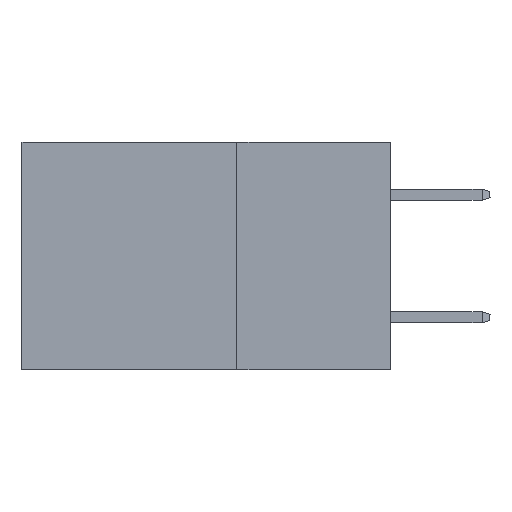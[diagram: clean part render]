
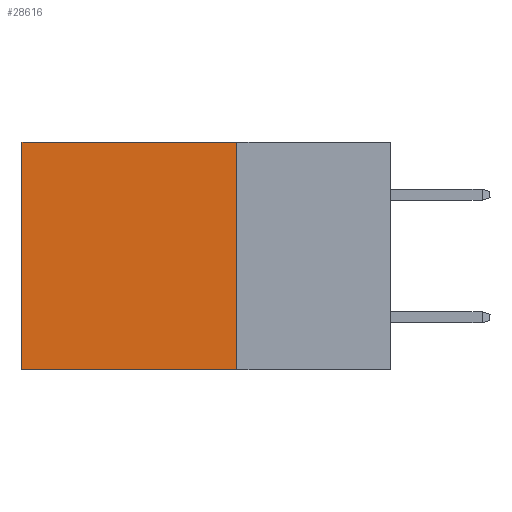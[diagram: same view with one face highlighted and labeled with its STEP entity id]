
A CAD part, left-side view. The second image highlights one B-rep face of the part: STEP entity #28616.
In plain terms, the highlighted planar face has unit normal (-1, 0, 0).
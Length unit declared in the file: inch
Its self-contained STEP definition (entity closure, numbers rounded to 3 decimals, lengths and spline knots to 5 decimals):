
#511 = CARTESIAN_POINT ( 'NONE',  ( 0.2875, 0.25, -0.37 ) ) ;
#609 = EDGE_CURVE ( 'NONE', #9454, #39162, #10498, .T. ) ;
#1040 = CARTESIAN_POINT ( 'NONE',  ( 0.2875, 0.6, 0. ) ) ;
#2229 = EDGE_LOOP ( 'NONE', ( #10578, #40993, #29764, #19286 ) ) ;
#2467 = VECTOR ( 'NONE', #25407, 39.37008 ) ;
#3616 = CARTESIAN_POINT ( 'NONE',  ( 0.2875, 0.25, -0.37 ) ) ;
#4548 = DIRECTION ( 'NONE',  ( 0., 1., 0. ) ) ;
#6862 = CARTESIAN_POINT ( 'NONE',  ( 0.2875, 0.25, 0. ) ) ;
#7890 = DIRECTION ( 'NONE',  ( 1., 0., 0. ) ) ;
#8518 = CARTESIAN_POINT ( 'NONE',  ( 0.2875, 0.6, 0. ) ) ;
#9454 = VERTEX_POINT ( 'NONE', #6862 ) ;
#9918 = VECTOR ( 'NONE', #38127, 39.37008 ) ;
#10498 = LINE ( 'NONE', #29094, #2467 ) ;
#10578 = ORIENTED_EDGE ( 'NONE', *, *, #25191, .T. ) ;
#10854 = DIRECTION ( 'NONE',  ( 0., 0., -1. ) ) ;
#13665 = VERTEX_POINT ( 'NONE', #8518 ) ;
#15408 = CARTESIAN_POINT ( 'NONE',  ( 0.2875, 0.6, -0.37 ) ) ;
#15564 = EDGE_CURVE ( 'NONE', #39162, #37660, #29697, .T. ) ;
#17108 = PLANE ( 'NONE',  #24430 ) ;
#19286 = ORIENTED_EDGE ( 'NONE', *, *, #36505, .T. ) ;
#22253 = VECTOR ( 'NONE', #27619, 39.37008 ) ;
#22520 = VECTOR ( 'NONE', #4548, 39.37008 ) ;
#22736 = LINE ( 'NONE', #1040, #9918 ) ;
#24430 = AXIS2_PLACEMENT_3D ( 'NONE', #34225, #7890, #10854 ) ;
#25191 = EDGE_CURVE ( 'NONE', #13665, #37660, #22736, .T. ) ;
#25407 = DIRECTION ( 'NONE',  ( 0., 0., -1. ) ) ;
#27619 = DIRECTION ( 'NONE',  ( 0., 1., 0. ) ) ;
#28345 = LINE ( 'NONE', #38471, #22520 ) ;
#28616 = ADVANCED_FACE ( 'NONE', ( #29114 ), #17108, .F. ) ;
#29094 = CARTESIAN_POINT ( 'NONE',  ( 0.2875, 0.25, 0. ) ) ;
#29114 = FACE_OUTER_BOUND ( 'NONE', #2229, .T. ) ;
#29697 = LINE ( 'NONE', #511, #22253 ) ;
#29764 = ORIENTED_EDGE ( 'NONE', *, *, #609, .F. ) ;
#34225 = CARTESIAN_POINT ( 'NONE',  ( 0.2875, 0.25, 0. ) ) ;
#36505 = EDGE_CURVE ( 'NONE', #9454, #13665, #28345, .T. ) ;
#37660 = VERTEX_POINT ( 'NONE', #15408 ) ;
#38127 = DIRECTION ( 'NONE',  ( 0., 0., -1. ) ) ;
#38471 = CARTESIAN_POINT ( 'NONE',  ( 0.2875, 0.25, 0. ) ) ;
#39162 = VERTEX_POINT ( 'NONE', #3616 ) ;
#40993 = ORIENTED_EDGE ( 'NONE', *, *, #15564, .F. ) ;
